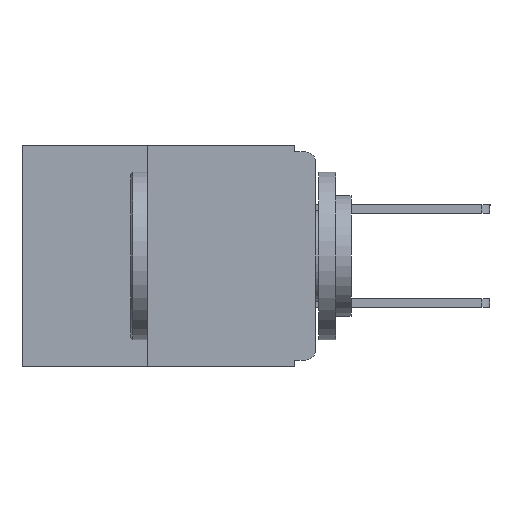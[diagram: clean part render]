
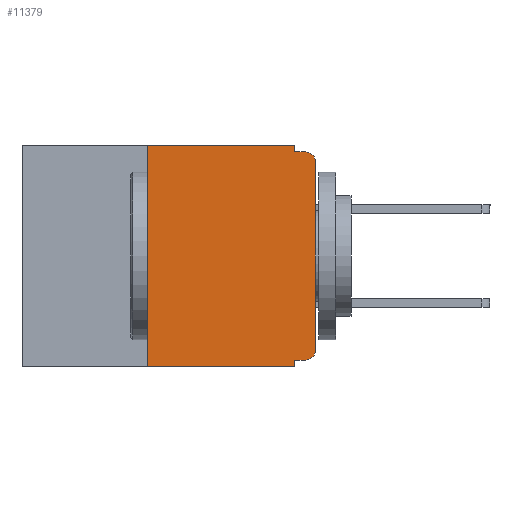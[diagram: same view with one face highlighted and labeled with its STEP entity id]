
A CAD part, left-side view. The second image highlights one B-rep face of the part: STEP entity #11379.
In plain terms, the highlighted planar face has unit normal (-1, 0, 0).
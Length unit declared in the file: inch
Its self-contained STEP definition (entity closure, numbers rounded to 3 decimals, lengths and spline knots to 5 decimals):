
#126 = CIRCLE ( 'NONE', #1049, 0.015 ) ;
#128 = EDGE_CURVE ( 'NONE', #13505, #3864, #10349, .T. ) ;
#559 = CARTESIAN_POINT ( 'NONE',  ( 0., 0., -0.01 ) ) ;
#782 = CARTESIAN_POINT ( 'NONE',  ( 0., 0.031, 0. ) ) ;
#812 = EDGE_CURVE ( 'NONE', #1517, #13099, #3289, .T. ) ;
#1012 = VECTOR ( 'NONE', #3323, 39.37008 ) ;
#1049 = AXIS2_PLACEMENT_3D ( 'NONE', #2023, #1973, #3741 ) ;
#1517 = VERTEX_POINT ( 'NONE', #1654 ) ;
#1615 = LINE ( 'NONE', #2227, #4166 ) ;
#1654 = CARTESIAN_POINT ( 'NONE',  ( 0., 0.031, -0.32 ) ) ;
#1663 = EDGE_CURVE ( 'NONE', #5844, #13099, #4261, .T. ) ;
#1772 = CARTESIAN_POINT ( 'NONE',  ( 0., 0.25, 0. ) ) ;
#1973 = DIRECTION ( 'NONE',  ( -1., 0., 0. ) ) ;
#2023 = CARTESIAN_POINT ( 'NONE',  ( 0., 0.015, -0.305 ) ) ;
#2075 = CARTESIAN_POINT ( 'NONE',  ( 0., 0., 0. ) ) ;
#2227 = CARTESIAN_POINT ( 'NONE',  ( 0., 0., -0.32 ) ) ;
#2651 = AXIS2_PLACEMENT_3D ( 'NONE', #2728, #10407, #3801 ) ;
#2728 = CARTESIAN_POINT ( 'NONE',  ( 0., 0.015, -0.025 ) ) ;
#2850 = CARTESIAN_POINT ( 'NONE',  ( 0., 0.25, -0.33 ) ) ;
#2869 = VERTEX_POINT ( 'NONE', #1772 ) ;
#3289 = LINE ( 'NONE', #9983, #12395 ) ;
#3323 = DIRECTION ( 'NONE',  ( 0., -1., 0. ) ) ;
#3358 = CIRCLE ( 'NONE', #2651, 0.015 ) ;
#3566 = CARTESIAN_POINT ( 'NONE',  ( 0., 0., -0.025 ) ) ;
#3741 = DIRECTION ( 'NONE',  ( 0., 0., -1. ) ) ;
#3801 = DIRECTION ( 'NONE',  ( 0., 0., -1. ) ) ;
#3864 = VERTEX_POINT ( 'NONE', #3566 ) ;
#3866 = VECTOR ( 'NONE', #7326, 39.37008 ) ;
#3871 = CARTESIAN_POINT ( 'NONE',  ( 0., 0.437, 0. ) ) ;
#3875 = DIRECTION ( 'NONE',  ( 0., 0., 1. ) ) ;
#3932 = CARTESIAN_POINT ( 'NONE',  ( 0., 0.031, -0.33 ) ) ;
#4065 = VECTOR ( 'NONE', #8315, 39.37008 ) ;
#4107 = FACE_OUTER_BOUND ( 'NONE', #4772, .T. ) ;
#4166 = VECTOR ( 'NONE', #8775, 39.37008 ) ;
#4167 = ORIENTED_EDGE ( 'NONE', *, *, #812, .F. ) ;
#4261 = LINE ( 'NONE', #10546, #1012 ) ;
#4532 = VECTOR ( 'NONE', #3875, 39.37008 ) ;
#4772 = EDGE_LOOP ( 'NONE', ( #5754, #6839, #5282, #12228, #13573, #12407, #11580, #4167, #5163, #6546 ) ) ;
#5025 = CARTESIAN_POINT ( 'NONE',  ( 0., 0.437, 0. ) ) ;
#5136 = VECTOR ( 'NONE', #6817, 39.37008 ) ;
#5163 = ORIENTED_EDGE ( 'NONE', *, *, #9047, .F. ) ;
#5282 = ORIENTED_EDGE ( 'NONE', *, *, #12480, .F. ) ;
#5578 = EDGE_CURVE ( 'NONE', #6126, #13505, #126, .T. ) ;
#5754 = ORIENTED_EDGE ( 'NONE', *, *, #128, .T. ) ;
#5834 = VERTEX_POINT ( 'NONE', #782 ) ;
#5844 = VERTEX_POINT ( 'NONE', #11455 ) ;
#5971 = DIRECTION ( 'NONE',  ( 0., 0., -1. ) ) ;
#6126 = VERTEX_POINT ( 'NONE', #9702 ) ;
#6135 = DIRECTION ( 'NONE',  ( 0., 0., -1. ) ) ;
#6546 = ORIENTED_EDGE ( 'NONE', *, *, #5578, .T. ) ;
#6813 = CARTESIAN_POINT ( 'NONE',  ( 0., 0., -0.305 ) ) ;
#6817 = DIRECTION ( 'NONE',  ( 0., 0., 1. ) ) ;
#6839 = ORIENTED_EDGE ( 'NONE', *, *, #13727, .T. ) ;
#7083 = VERTEX_POINT ( 'NONE', #10739 ) ;
#7319 = LINE ( 'NONE', #559, #4065 ) ;
#7326 = DIRECTION ( 'NONE',  ( 0., 0., -1. ) ) ;
#7936 = VERTEX_POINT ( 'NONE', #10195 ) ;
#8315 = DIRECTION ( 'NONE',  ( 0., -1., 0. ) ) ;
#8773 = AXIS2_PLACEMENT_3D ( 'NONE', #5025, #12778, #6135 ) ;
#8775 = DIRECTION ( 'NONE',  ( 0., 1., 0. ) ) ;
#8949 = LINE ( 'NONE', #3871, #10876 ) ;
#9047 = EDGE_CURVE ( 'NONE', #6126, #1517, #1615, .T. ) ;
#9702 = CARTESIAN_POINT ( 'NONE',  ( 0., 0.015, -0.32 ) ) ;
#9983 = CARTESIAN_POINT ( 'NONE',  ( 0., 0.031, -0.33 ) ) ;
#10195 = CARTESIAN_POINT ( 'NONE',  ( 0., 0.031, -0.01 ) ) ;
#10349 = LINE ( 'NONE', #2075, #5136 ) ;
#10407 = DIRECTION ( 'NONE',  ( -1., 0., 0. ) ) ;
#10422 = LINE ( 'NONE', #2850, #4532 ) ;
#10539 = EDGE_CURVE ( 'NONE', #2869, #5834, #8949, .T. ) ;
#10546 = CARTESIAN_POINT ( 'NONE',  ( 0., 0.437, -0.33 ) ) ;
#10628 = CARTESIAN_POINT ( 'NONE',  ( 0., 0.031, 0. ) ) ;
#10739 = CARTESIAN_POINT ( 'NONE',  ( 0., 0.015, -0.01 ) ) ;
#10876 = VECTOR ( 'NONE', #11587, 39.37008 ) ;
#11379 = ADVANCED_FACE ( 'NONE', ( #4107 ), #12726, .F. ) ;
#11455 = CARTESIAN_POINT ( 'NONE',  ( 0., 0.25, -0.33 ) ) ;
#11580 = ORIENTED_EDGE ( 'NONE', *, *, #1663, .T. ) ;
#11587 = DIRECTION ( 'NONE',  ( 0., -1., 0. ) ) ;
#12228 = ORIENTED_EDGE ( 'NONE', *, *, #13148, .F. ) ;
#12395 = VECTOR ( 'NONE', #5971, 39.37008 ) ;
#12407 = ORIENTED_EDGE ( 'NONE', *, *, #13076, .F. ) ;
#12480 = EDGE_CURVE ( 'NONE', #7936, #7083, #7319, .T. ) ;
#12654 = LINE ( 'NONE', #10628, #3866 ) ;
#12726 = PLANE ( 'NONE',  #8773 ) ;
#12778 = DIRECTION ( 'NONE',  ( 1., 0., 0. ) ) ;
#13076 = EDGE_CURVE ( 'NONE', #5844, #2869, #10422, .T. ) ;
#13099 = VERTEX_POINT ( 'NONE', #3932 ) ;
#13148 = EDGE_CURVE ( 'NONE', #5834, #7936, #12654, .T. ) ;
#13505 = VERTEX_POINT ( 'NONE', #6813 ) ;
#13573 = ORIENTED_EDGE ( 'NONE', *, *, #10539, .F. ) ;
#13727 = EDGE_CURVE ( 'NONE', #3864, #7083, #3358, .T. ) ;
